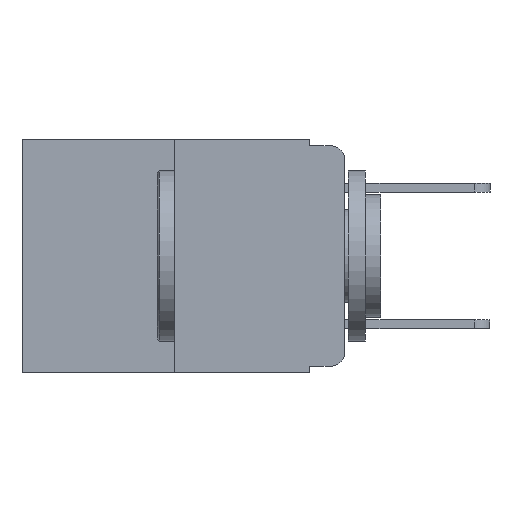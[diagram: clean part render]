
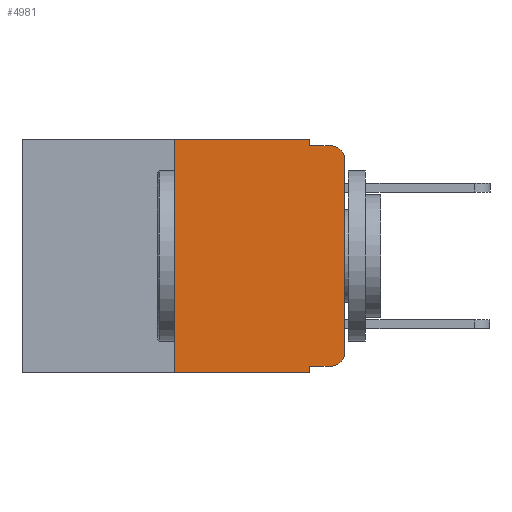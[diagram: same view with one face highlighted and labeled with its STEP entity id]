
A CAD part, left-side view. The second image highlights one B-rep face of the part: STEP entity #4981.
In plain terms, the highlighted planar face has unit normal (-1, 0, 0).
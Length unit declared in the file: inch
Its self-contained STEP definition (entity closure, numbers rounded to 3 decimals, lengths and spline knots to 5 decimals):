
#113 = EDGE_CURVE ( 'NONE', #14174, #19996, #2973, .T. ) ;
#161 = DIRECTION ( 'NONE',  ( -1., 0., 0. ) ) ;
#195 = AXIS2_PLACEMENT_3D ( 'NONE', #19311, #6606, #6578 ) ;
#548 = CARTESIAN_POINT ( 'NONE',  ( 0., 0.25, 0. ) ) ;
#836 = DIRECTION ( 'NONE',  ( 0., 0., -1. ) ) ;
#1113 = DIRECTION ( 'NONE',  ( 0., 0., -1. ) ) ;
#1237 = CARTESIAN_POINT ( 'NONE',  ( 0., 0.473, 0. ) ) ;
#1324 = CARTESIAN_POINT ( 'NONE',  ( 0., 0.051, 0. ) ) ;
#1353 = VERTEX_POINT ( 'NONE', #21943 ) ;
#2042 = LINE ( 'NONE', #1237, #17061 ) ;
#2655 = VECTOR ( 'NONE', #6788, 39.37008 ) ;
#2733 = DIRECTION ( 'NONE',  ( 0., -1., 0. ) ) ;
#2852 = EDGE_CURVE ( 'NONE', #1353, #22010, #22862, .T. ) ;
#2973 = LINE ( 'NONE', #548, #6758 ) ;
#2981 = ORIENTED_EDGE ( 'NONE', *, *, #20132, .T. ) ;
#3028 = CIRCLE ( 'NONE', #7385, 0.02 ) ;
#3301 = ORIENTED_EDGE ( 'NONE', *, *, #5980, .T. ) ;
#3444 = EDGE_CURVE ( 'NONE', #11995, #17747, #3028, .T. ) ;
#4118 = DIRECTION ( 'NONE',  ( 0., 0., 1. ) ) ;
#4175 = ORIENTED_EDGE ( 'NONE', *, *, #20482, .F. ) ;
#4981 = ADVANCED_FACE ( 'NONE', ( #8138 ), #9610, .F. ) ;
#5434 = VERTEX_POINT ( 'NONE', #8410 ) ;
#5494 = EDGE_CURVE ( 'NONE', #7957, #5434, #8118, .T. ) ;
#5822 = CARTESIAN_POINT ( 'NONE',  ( 0., 0.02, -0.333 ) ) ;
#5980 = EDGE_CURVE ( 'NONE', #14174, #19182, #16504, .T. ) ;
#6578 = DIRECTION ( 'NONE',  ( 0., 0., -1. ) ) ;
#6606 = DIRECTION ( 'NONE',  ( 1., 0., 0. ) ) ;
#6758 = VECTOR ( 'NONE', #4118, 39.37008 ) ;
#6788 = DIRECTION ( 'NONE',  ( 0., 0., -1. ) ) ;
#6867 = CARTESIAN_POINT ( 'NONE',  ( 0., 0.02, -0.01 ) ) ;
#7194 = DIRECTION ( 'NONE',  ( 0., 0., -1. ) ) ;
#7385 = AXIS2_PLACEMENT_3D ( 'NONE', #13366, #161, #1113 ) ;
#7431 = CARTESIAN_POINT ( 'NONE',  ( 0., 0.25, -0.343 ) ) ;
#7506 = VECTOR ( 'NONE', #2733, 39.37008 ) ;
#7939 = CARTESIAN_POINT ( 'NONE',  ( 0., 0.25, 0. ) ) ;
#7957 = VERTEX_POINT ( 'NONE', #8412 ) ;
#8118 = LINE ( 'NONE', #10300, #17105 ) ;
#8138 = FACE_OUTER_BOUND ( 'NONE', #17791, .T. ) ;
#8375 = DIRECTION ( 'NONE',  ( 0., -1., 0. ) ) ;
#8410 = CARTESIAN_POINT ( 'NONE',  ( 0., 0.051, -0.01 ) ) ;
#8412 = CARTESIAN_POINT ( 'NONE',  ( 0., 0.051, 0. ) ) ;
#8683 = LINE ( 'NONE', #1324, #2655 ) ;
#9561 = ORIENTED_EDGE ( 'NONE', *, *, #113, .F. ) ;
#9610 = PLANE ( 'NONE',  #195 ) ;
#10145 = CARTESIAN_POINT ( 'NONE',  ( 0., 0.051, -0.01 ) ) ;
#10300 = CARTESIAN_POINT ( 'NONE',  ( 0., 0.051, 0. ) ) ;
#10832 = CIRCLE ( 'NONE', #12187, 0.02 ) ;
#10954 = ORIENTED_EDGE ( 'NONE', *, *, #19561, .F. ) ;
#11650 = DIRECTION ( 'NONE',  ( -1., 0., 0. ) ) ;
#11995 = VERTEX_POINT ( 'NONE', #18783 ) ;
#12187 = AXIS2_PLACEMENT_3D ( 'NONE', #22510, #11650, #836 ) ;
#12722 = CARTESIAN_POINT ( 'NONE',  ( 0., 0.051, -0.343 ) ) ;
#13090 = ORIENTED_EDGE ( 'NONE', *, *, #3444, .T. ) ;
#13366 = CARTESIAN_POINT ( 'NONE',  ( 0., 0.02, -0.03 ) ) ;
#13503 = VECTOR ( 'NONE', #8375, 39.37008 ) ;
#13574 = VECTOR ( 'NONE', #19102, 39.37008 ) ;
#13809 = DIRECTION ( 'NONE',  ( 0., -1., 0. ) ) ;
#14174 = VERTEX_POINT ( 'NONE', #7431 ) ;
#14312 = ORIENTED_EDGE ( 'NONE', *, *, #20338, .T. ) ;
#14336 = VECTOR ( 'NONE', #15578, 39.37008 ) ;
#15159 = ORIENTED_EDGE ( 'NONE', *, *, #5494, .F. ) ;
#15377 = CARTESIAN_POINT ( 'NONE',  ( 0., 0.473, -0.343 ) ) ;
#15571 = EDGE_CURVE ( 'NONE', #5434, #17747, #18412, .T. ) ;
#15578 = DIRECTION ( 'NONE',  ( 0., -1., 0. ) ) ;
#16337 = ORIENTED_EDGE ( 'NONE', *, *, #2852, .T. ) ;
#16504 = LINE ( 'NONE', #15377, #7506 ) ;
#17061 = VECTOR ( 'NONE', #13809, 39.37008 ) ;
#17105 = VECTOR ( 'NONE', #7194, 39.37008 ) ;
#17281 = CARTESIAN_POINT ( 'NONE',  ( 0., 0., 0. ) ) ;
#17747 = VERTEX_POINT ( 'NONE', #6867 ) ;
#17791 = EDGE_LOOP ( 'NONE', ( #2981, #13090, #21430, #15159, #4175, #9561, #3301, #10954, #16337, #14312 ) ) ;
#18412 = LINE ( 'NONE', #10145, #13503 ) ;
#18779 = CARTESIAN_POINT ( 'NONE',  ( 0., 0.051, -0.333 ) ) ;
#18783 = CARTESIAN_POINT ( 'NONE',  ( 0., 0., -0.03 ) ) ;
#19063 = LINE ( 'NONE', #17281, #13574 ) ;
#19102 = DIRECTION ( 'NONE',  ( 0., 0., 1. ) ) ;
#19182 = VERTEX_POINT ( 'NONE', #12722 ) ;
#19311 = CARTESIAN_POINT ( 'NONE',  ( 0., 0.473, 0. ) ) ;
#19561 = EDGE_CURVE ( 'NONE', #1353, #19182, #8683, .T. ) ;
#19996 = VERTEX_POINT ( 'NONE', #7939 ) ;
#20132 = EDGE_CURVE ( 'NONE', #20843, #11995, #19063, .T. ) ;
#20296 = CARTESIAN_POINT ( 'NONE',  ( 0., 0., -0.313 ) ) ;
#20338 = EDGE_CURVE ( 'NONE', #22010, #20843, #10832, .T. ) ;
#20482 = EDGE_CURVE ( 'NONE', #19996, #7957, #2042, .T. ) ;
#20843 = VERTEX_POINT ( 'NONE', #20296 ) ;
#21430 = ORIENTED_EDGE ( 'NONE', *, *, #15571, .F. ) ;
#21943 = CARTESIAN_POINT ( 'NONE',  ( 0., 0.051, -0.333 ) ) ;
#22010 = VERTEX_POINT ( 'NONE', #5822 ) ;
#22510 = CARTESIAN_POINT ( 'NONE',  ( 0., 0.02, -0.313 ) ) ;
#22862 = LINE ( 'NONE', #18779, #14336 ) ;
